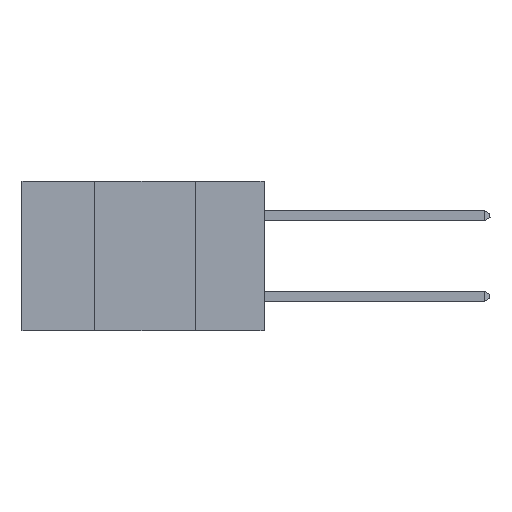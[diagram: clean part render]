
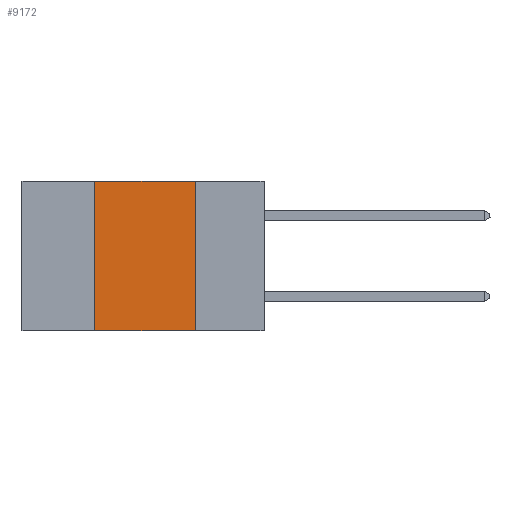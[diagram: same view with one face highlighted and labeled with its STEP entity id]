
A CAD part, left-side view. The second image highlights one B-rep face of the part: STEP entity #9172.
In plain terms, the highlighted planar face has unit normal (-1, 0, 0).
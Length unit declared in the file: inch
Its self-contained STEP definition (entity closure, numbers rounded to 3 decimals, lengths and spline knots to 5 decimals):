
#40 = ORIENTED_EDGE ( 'NONE', *, *, #1206, .F. ) ;
#166 = VECTOR ( 'NONE', #6867, 39.37008 ) ;
#323 = CARTESIAN_POINT ( 'NONE',  ( 0., 0.17, 0. ) ) ;
#857 = FACE_OUTER_BOUND ( 'NONE', #5877, .T. ) ;
#934 = CARTESIAN_POINT ( 'NONE',  ( 0., 0.17, 0. ) ) ;
#955 = CARTESIAN_POINT ( 'NONE',  ( 0., 0.42, 0. ) ) ;
#1206 = EDGE_CURVE ( 'NONE', #4262, #12067, #1995, .T. ) ;
#1606 = AXIS2_PLACEMENT_3D ( 'NONE', #9467, #11600, #10701 ) ;
#1995 = LINE ( 'NONE', #10397, #7910 ) ;
#2154 = CARTESIAN_POINT ( 'NONE',  ( 0., 0.17, -0.37 ) ) ;
#3140 = VECTOR ( 'NONE', #8477, 39.37008 ) ;
#3387 = EDGE_CURVE ( 'NONE', #4262, #12231, #9728, .T. ) ;
#3777 = ORIENTED_EDGE ( 'NONE', *, *, #13147, .F. ) ;
#4079 = CARTESIAN_POINT ( 'NONE',  ( 0., 0.42, -0.37 ) ) ;
#4259 = PLANE ( 'NONE',  #1606 ) ;
#4262 = VERTEX_POINT ( 'NONE', #4079 ) ;
#5523 = LINE ( 'NONE', #934, #3140 ) ;
#5877 = EDGE_LOOP ( 'NONE', ( #10546, #3777, #40, #9968 ) ) ;
#6127 = DIRECTION ( 'NONE',  ( 0., -1., 0. ) ) ;
#6166 = EDGE_CURVE ( 'NONE', #12284, #12231, #5523, .T. ) ;
#6867 = DIRECTION ( 'NONE',  ( 0., -1., 0. ) ) ;
#7243 = LINE ( 'NONE', #13440, #166 ) ;
#7910 = VECTOR ( 'NONE', #10443, 39.37008 ) ;
#8033 = VECTOR ( 'NONE', #6127, 39.37008 ) ;
#8477 = DIRECTION ( 'NONE',  ( 0., 0., -1. ) ) ;
#9172 = ADVANCED_FACE ( 'NONE', ( #857 ), #4259, .F. ) ;
#9278 = CARTESIAN_POINT ( 'NONE',  ( 0., 0.6, -0.37 ) ) ;
#9467 = CARTESIAN_POINT ( 'NONE',  ( 0., 0.6, 0. ) ) ;
#9728 = LINE ( 'NONE', #9278, #8033 ) ;
#9968 = ORIENTED_EDGE ( 'NONE', *, *, #3387, .T. ) ;
#10397 = CARTESIAN_POINT ( 'NONE',  ( 0., 0.42, 0. ) ) ;
#10443 = DIRECTION ( 'NONE',  ( 0., 0., 1. ) ) ;
#10546 = ORIENTED_EDGE ( 'NONE', *, *, #6166, .F. ) ;
#10701 = DIRECTION ( 'NONE',  ( 0., 0., -1. ) ) ;
#11600 = DIRECTION ( 'NONE',  ( 1., 0., 0. ) ) ;
#12067 = VERTEX_POINT ( 'NONE', #955 ) ;
#12231 = VERTEX_POINT ( 'NONE', #2154 ) ;
#12284 = VERTEX_POINT ( 'NONE', #323 ) ;
#13147 = EDGE_CURVE ( 'NONE', #12067, #12284, #7243, .T. ) ;
#13440 = CARTESIAN_POINT ( 'NONE',  ( 0., 0.6, 0. ) ) ;
